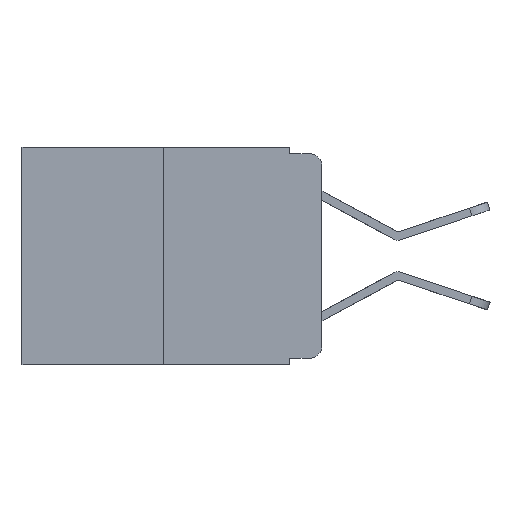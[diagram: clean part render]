
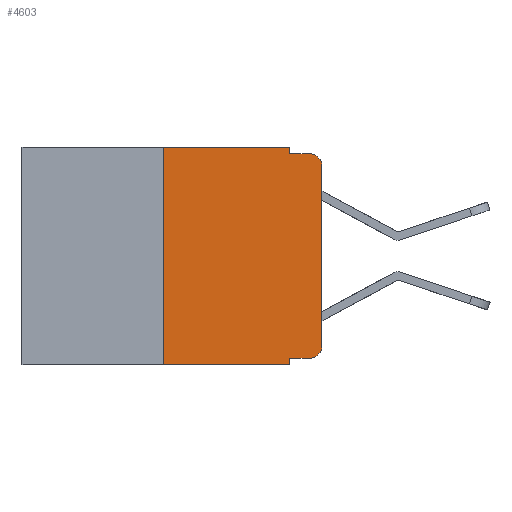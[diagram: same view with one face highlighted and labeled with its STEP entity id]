
A CAD part, left-side view. The second image highlights one B-rep face of the part: STEP entity #4603.
In plain terms, the highlighted planar face has unit normal (-1, 0, 0).
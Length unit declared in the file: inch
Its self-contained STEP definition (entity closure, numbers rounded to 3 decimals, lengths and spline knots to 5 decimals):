
#247 = CARTESIAN_POINT ( 'NONE',  ( 0., 0.051, -0.01 ) ) ;
#327 = CARTESIAN_POINT ( 'NONE',  ( 0., 0.051, 0. ) ) ;
#466 = CARTESIAN_POINT ( 'NONE',  ( 0., 0.25, -0.343 ) ) ;
#1063 = VERTEX_POINT ( 'NONE', #1653 ) ;
#1653 = CARTESIAN_POINT ( 'NONE',  ( 0., 0.051, -0.333 ) ) ;
#2450 = EDGE_CURVE ( 'NONE', #16067, #20995, #3637, .T. ) ;
#2474 = VECTOR ( 'NONE', #21328, 39.37008 ) ;
#2532 = CARTESIAN_POINT ( 'NONE',  ( 0., 0.02, -0.313 ) ) ;
#3171 = EDGE_CURVE ( 'NONE', #1063, #7241, #11182, .T. ) ;
#3211 = VERTEX_POINT ( 'NONE', #9545 ) ;
#3288 = EDGE_LOOP ( 'NONE', ( #20019, #15264, #9847, #3538, #20088, #6275, #9085, #14112, #11479, #8829 ) ) ;
#3297 = EDGE_CURVE ( 'NONE', #6819, #6330, #6599, .T. ) ;
#3378 = VECTOR ( 'NONE', #18589, 39.37008 ) ;
#3386 = VECTOR ( 'NONE', #18241, 39.37008 ) ;
#3449 = CARTESIAN_POINT ( 'NONE',  ( 0., 0.02, -0.333 ) ) ;
#3481 = CARTESIAN_POINT ( 'NONE',  ( 0., 0.051, -0.01 ) ) ;
#3538 = ORIENTED_EDGE ( 'NONE', *, *, #20817, .F. ) ;
#3637 = LINE ( 'NONE', #14695, #21247 ) ;
#4483 = DIRECTION ( 'NONE',  ( 0., -1., 0. ) ) ;
#4603 = ADVANCED_FACE ( 'NONE', ( #5314 ), #15516, .F. ) ;
#4903 = CARTESIAN_POINT ( 'NONE',  ( 0., 0., 0. ) ) ;
#5005 = LINE ( 'NONE', #11615, #3386 ) ;
#5136 = LINE ( 'NONE', #327, #3378 ) ;
#5314 = FACE_OUTER_BOUND ( 'NONE', #3288, .T. ) ;
#6275 = ORIENTED_EDGE ( 'NONE', *, *, #9973, .F. ) ;
#6330 = VERTEX_POINT ( 'NONE', #10161 ) ;
#6547 = CARTESIAN_POINT ( 'NONE',  ( 0., 0.051, -0.333 ) ) ;
#6599 = LINE ( 'NONE', #3481, #19907 ) ;
#6731 = DIRECTION ( 'NONE',  ( 0., 0., 1. ) ) ;
#6819 = VERTEX_POINT ( 'NONE', #247 ) ;
#7241 = VERTEX_POINT ( 'NONE', #10305 ) ;
#7339 = AXIS2_PLACEMENT_3D ( 'NONE', #2532, #9349, #20980 ) ;
#7696 = DIRECTION ( 'NONE',  ( 0., 0., -1. ) ) ;
#7994 = VECTOR ( 'NONE', #6731, 39.37008 ) ;
#8089 = EDGE_CURVE ( 'NONE', #1063, #18673, #14708, .T. ) ;
#8241 = VERTEX_POINT ( 'NONE', #466 ) ;
#8553 = CARTESIAN_POINT ( 'NONE',  ( 0., 0.25, 0. ) ) ;
#8829 = ORIENTED_EDGE ( 'NONE', *, *, #14007, .T. ) ;
#9085 = ORIENTED_EDGE ( 'NONE', *, *, #12705, .T. ) ;
#9349 = DIRECTION ( 'NONE',  ( -1., 0., 0. ) ) ;
#9525 = EDGE_CURVE ( 'NONE', #3211, #6330, #10342, .T. ) ;
#9545 = CARTESIAN_POINT ( 'NONE',  ( 0., 0., -0.03 ) ) ;
#9847 = ORIENTED_EDGE ( 'NONE', *, *, #3297, .F. ) ;
#9973 = EDGE_CURVE ( 'NONE', #8241, #16067, #5005, .T. ) ;
#10161 = CARTESIAN_POINT ( 'NONE',  ( 0., 0.02, -0.01 ) ) ;
#10305 = CARTESIAN_POINT ( 'NONE',  ( 0., 0.051, -0.343 ) ) ;
#10342 = CIRCLE ( 'NONE', #16250, 0.02 ) ;
#10443 = DIRECTION ( 'NONE',  ( -1., 0., 0. ) ) ;
#10473 = CIRCLE ( 'NONE', #7339, 0.02 ) ;
#11182 = LINE ( 'NONE', #19017, #14348 ) ;
#11479 = ORIENTED_EDGE ( 'NONE', *, *, #8089, .T. ) ;
#11615 = CARTESIAN_POINT ( 'NONE',  ( 0., 0.25, 0. ) ) ;
#11719 = DIRECTION ( 'NONE',  ( 0., -1., 0. ) ) ;
#11874 = DIRECTION ( 'NONE',  ( 0., -1., 0. ) ) ;
#11929 = CARTESIAN_POINT ( 'NONE',  ( 0., 0.473, 0. ) ) ;
#12181 = DIRECTION ( 'NONE',  ( 0., 0., -1. ) ) ;
#12705 = EDGE_CURVE ( 'NONE', #8241, #7241, #17513, .T. ) ;
#12746 = EDGE_CURVE ( 'NONE', #13316, #3211, #17932, .T. ) ;
#12823 = CARTESIAN_POINT ( 'NONE',  ( 0., 0.473, -0.343 ) ) ;
#13316 = VERTEX_POINT ( 'NONE', #14935 ) ;
#13537 = VECTOR ( 'NONE', #4483, 39.37008 ) ;
#13906 = CARTESIAN_POINT ( 'NONE',  ( 0., 0.051, 0. ) ) ;
#14007 = EDGE_CURVE ( 'NONE', #18673, #13316, #10473, .T. ) ;
#14112 = ORIENTED_EDGE ( 'NONE', *, *, #3171, .F. ) ;
#14348 = VECTOR ( 'NONE', #7696, 39.37008 ) ;
#14629 = AXIS2_PLACEMENT_3D ( 'NONE', #11929, #18769, #16933 ) ;
#14695 = CARTESIAN_POINT ( 'NONE',  ( 0., 0.473, 0. ) ) ;
#14708 = LINE ( 'NONE', #6547, #2474 ) ;
#14935 = CARTESIAN_POINT ( 'NONE',  ( 0., 0., -0.313 ) ) ;
#15264 = ORIENTED_EDGE ( 'NONE', *, *, #9525, .T. ) ;
#15516 = PLANE ( 'NONE',  #14629 ) ;
#16067 = VERTEX_POINT ( 'NONE', #8553 ) ;
#16250 = AXIS2_PLACEMENT_3D ( 'NONE', #20230, #10443, #12181 ) ;
#16933 = DIRECTION ( 'NONE',  ( 0., 0., -1. ) ) ;
#17513 = LINE ( 'NONE', #12823, #13537 ) ;
#17932 = LINE ( 'NONE', #4903, #7994 ) ;
#18241 = DIRECTION ( 'NONE',  ( 0., 0., 1. ) ) ;
#18589 = DIRECTION ( 'NONE',  ( 0., 0., -1. ) ) ;
#18673 = VERTEX_POINT ( 'NONE', #3449 ) ;
#18769 = DIRECTION ( 'NONE',  ( 1., 0., 0. ) ) ;
#19017 = CARTESIAN_POINT ( 'NONE',  ( 0., 0.051, 0. ) ) ;
#19907 = VECTOR ( 'NONE', #11719, 39.37008 ) ;
#20019 = ORIENTED_EDGE ( 'NONE', *, *, #12746, .T. ) ;
#20088 = ORIENTED_EDGE ( 'NONE', *, *, #2450, .F. ) ;
#20230 = CARTESIAN_POINT ( 'NONE',  ( 0., 0.02, -0.03 ) ) ;
#20817 = EDGE_CURVE ( 'NONE', #20995, #6819, #5136, .T. ) ;
#20980 = DIRECTION ( 'NONE',  ( 0., 0., -1. ) ) ;
#20995 = VERTEX_POINT ( 'NONE', #13906 ) ;
#21247 = VECTOR ( 'NONE', #11874, 39.37008 ) ;
#21328 = DIRECTION ( 'NONE',  ( 0., -1., 0. ) ) ;
